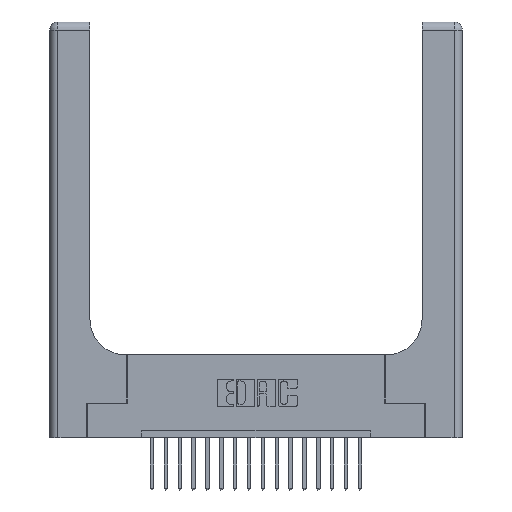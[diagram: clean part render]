
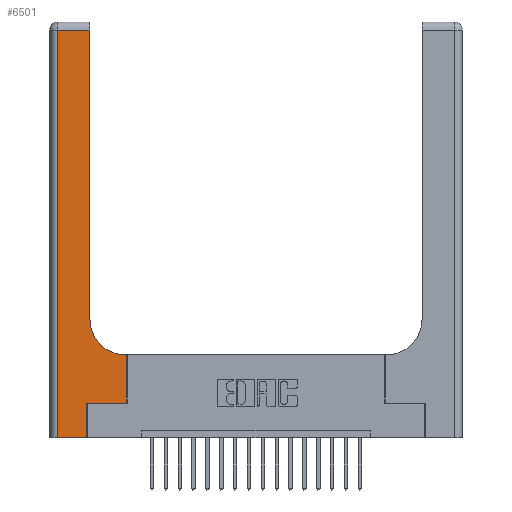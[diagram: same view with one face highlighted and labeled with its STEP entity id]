
A CAD part, top view. The second image highlights one B-rep face of the part: STEP entity #6501.
In plain terms, the highlighted planar face has unit normal (0, 0, 1).
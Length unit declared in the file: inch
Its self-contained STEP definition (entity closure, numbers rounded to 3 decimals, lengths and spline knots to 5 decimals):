
#95 = VERTEX_POINT ( 'NONE', #19034 ) ;
#158 = DIRECTION ( 'NONE',  ( -1., 0., 0. ) ) ;
#444 = CARTESIAN_POINT ( 'NONE',  ( 0.269, 0., 0.37 ) ) ;
#546 = CARTESIAN_POINT ( 'NONE',  ( 0.2915, 3., 0.37 ) ) ;
#1024 = VECTOR ( 'NONE', #158, 39.37008 ) ;
#1032 = CARTESIAN_POINT ( 'NONE',  ( 0.2915, 0.85, 0.37 ) ) ;
#1475 = ORIENTED_EDGE ( 'NONE', *, *, #8711, .T. ) ;
#1686 = ORIENTED_EDGE ( 'NONE', *, *, #7759, .T. ) ;
#2068 = FACE_OUTER_BOUND ( 'NONE', #8685, .T. ) ;
#2719 = AXIS2_PLACEMENT_3D ( 'NONE', #12749, #17224, #14304 ) ;
#2762 = LINE ( 'NONE', #13404, #16532 ) ;
#2789 = CARTESIAN_POINT ( 'NONE',  ( 0.5415, 0.6, 0.37 ) ) ;
#2918 = CARTESIAN_POINT ( 'NONE',  ( 0.5415, 0.85, 0.37 ) ) ;
#3117 = VERTEX_POINT ( 'NONE', #12306 ) ;
#3133 = VECTOR ( 'NONE', #9687, 39.37008 ) ;
#3335 = LINE ( 'NONE', #9177, #6647 ) ;
#3386 = AXIS2_PLACEMENT_3D ( 'NONE', #2918, #17175, #6153 ) ;
#3510 = DIRECTION ( 'NONE',  ( 0., 1., 0. ) ) ;
#3518 = PLANE ( 'NONE',  #2719 ) ;
#3898 = LINE ( 'NONE', #11207, #3133 ) ;
#3963 = DIRECTION ( 'NONE',  ( 0., 1., 0. ) ) ;
#4775 = DIRECTION ( 'NONE',  ( -1., 0., 0. ) ) ;
#5106 = EDGE_CURVE ( 'NONE', #7415, #11851, #3898, .T. ) ;
#5336 = CIRCLE ( 'NONE', #3386, 0.25 ) ;
#6153 = DIRECTION ( 'NONE',  ( 1., 0., 0. ) ) ;
#6501 = ADVANCED_FACE ( 'NONE', ( #2068 ), #3518, .F. ) ;
#6611 = CARTESIAN_POINT ( 'NONE',  ( 0.06, 2.94, 0.37 ) ) ;
#6647 = VECTOR ( 'NONE', #4775, 39.37008 ) ;
#6705 = CARTESIAN_POINT ( 'NONE',  ( 0., 2.94, 0.37 ) ) ;
#7244 = ORIENTED_EDGE ( 'NONE', *, *, #17004, .T. ) ;
#7301 = LINE ( 'NONE', #19355, #13775 ) ;
#7415 = VERTEX_POINT ( 'NONE', #444 ) ;
#7759 = EDGE_CURVE ( 'NONE', #95, #15391, #8581, .T. ) ;
#8209 = DIRECTION ( 'NONE',  ( 1., 0., 0. ) ) ;
#8247 = LINE ( 'NONE', #546, #17217 ) ;
#8475 = EDGE_CURVE ( 'NONE', #9183, #3117, #7301, .T. ) ;
#8581 = LINE ( 'NONE', #6705, #1024 ) ;
#8685 = EDGE_LOOP ( 'NONE', ( #11698, #1686, #1475, #19998, #18687, #7244, #13579, #10655, #15190 ) ) ;
#8687 = CARTESIAN_POINT ( 'NONE',  ( 0.269, 0.25, 0.37 ) ) ;
#8711 = EDGE_CURVE ( 'NONE', #15391, #16262, #12767, .T. ) ;
#8769 = VECTOR ( 'NONE', #15438, 39.37008 ) ;
#9177 = CARTESIAN_POINT ( 'NONE',  ( 0.2915, 0.6, 0.37 ) ) ;
#9183 = VERTEX_POINT ( 'NONE', #10874 ) ;
#9687 = DIRECTION ( 'NONE',  ( 0., 1., 0. ) ) ;
#10197 = EDGE_CURVE ( 'NONE', #16262, #7415, #17706, .T. ) ;
#10655 = ORIENTED_EDGE ( 'NONE', *, *, #17845, .T. ) ;
#10850 = CARTESIAN_POINT ( 'NONE',  ( 0.06, 0., 0.37 ) ) ;
#10874 = CARTESIAN_POINT ( 'NONE',  ( 0.5585, 0.25, 0.37 ) ) ;
#11207 = CARTESIAN_POINT ( 'NONE',  ( 0.269, 0., 0.37 ) ) ;
#11520 = EDGE_CURVE ( 'NONE', #17834, #95, #8247, .T. ) ;
#11698 = ORIENTED_EDGE ( 'NONE', *, *, #11520, .T. ) ;
#11851 = VERTEX_POINT ( 'NONE', #8687 ) ;
#12306 = CARTESIAN_POINT ( 'NONE',  ( 0.5585, 0.6, 0.37 ) ) ;
#12749 = CARTESIAN_POINT ( 'NONE',  ( 0., 3., 0.37 ) ) ;
#12767 = LINE ( 'NONE', #17181, #8769 ) ;
#13277 = VERTEX_POINT ( 'NONE', #2789 ) ;
#13404 = CARTESIAN_POINT ( 'NONE',  ( 0.269, 0.25, 0.37 ) ) ;
#13579 = ORIENTED_EDGE ( 'NONE', *, *, #8475, .T. ) ;
#13775 = VECTOR ( 'NONE', #3510, 39.37008 ) ;
#14304 = DIRECTION ( 'NONE',  ( -1., 0., 0. ) ) ;
#15190 = ORIENTED_EDGE ( 'NONE', *, *, #18369, .T. ) ;
#15391 = VERTEX_POINT ( 'NONE', #6611 ) ;
#15438 = DIRECTION ( 'NONE',  ( 0., -1., 0. ) ) ;
#16262 = VERTEX_POINT ( 'NONE', #10850 ) ;
#16289 = CARTESIAN_POINT ( 'NONE',  ( 0., 0., 0.37 ) ) ;
#16532 = VECTOR ( 'NONE', #16820, 39.37008 ) ;
#16820 = DIRECTION ( 'NONE',  ( 1., 0., 0. ) ) ;
#17004 = EDGE_CURVE ( 'NONE', #11851, #9183, #2762, .T. ) ;
#17175 = DIRECTION ( 'NONE',  ( 0., 0., -1. ) ) ;
#17181 = CARTESIAN_POINT ( 'NONE',  ( 0.06, 3., 0.37 ) ) ;
#17217 = VECTOR ( 'NONE', #3963, 39.37008 ) ;
#17224 = DIRECTION ( 'NONE',  ( 0., 0., -1. ) ) ;
#17706 = LINE ( 'NONE', #16289, #19972 ) ;
#17834 = VERTEX_POINT ( 'NONE', #1032 ) ;
#17845 = EDGE_CURVE ( 'NONE', #3117, #13277, #3335, .T. ) ;
#18369 = EDGE_CURVE ( 'NONE', #13277, #17834, #5336, .T. ) ;
#18687 = ORIENTED_EDGE ( 'NONE', *, *, #5106, .T. ) ;
#19034 = CARTESIAN_POINT ( 'NONE',  ( 0.2915, 2.94, 0.37 ) ) ;
#19355 = CARTESIAN_POINT ( 'NONE',  ( 0.5585, 0.25, 0.37 ) ) ;
#19972 = VECTOR ( 'NONE', #8209, 39.37008 ) ;
#19998 = ORIENTED_EDGE ( 'NONE', *, *, #10197, .T. ) ;
